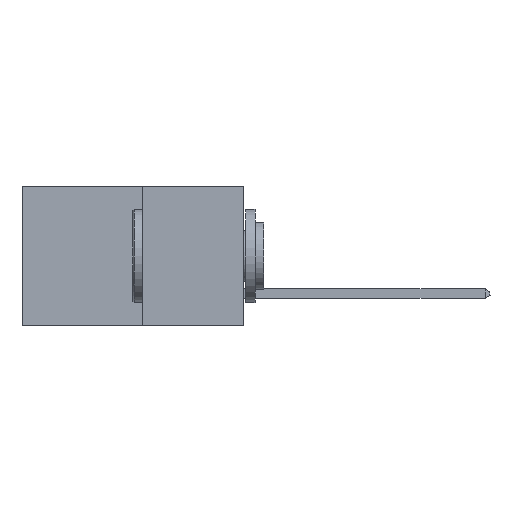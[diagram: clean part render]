
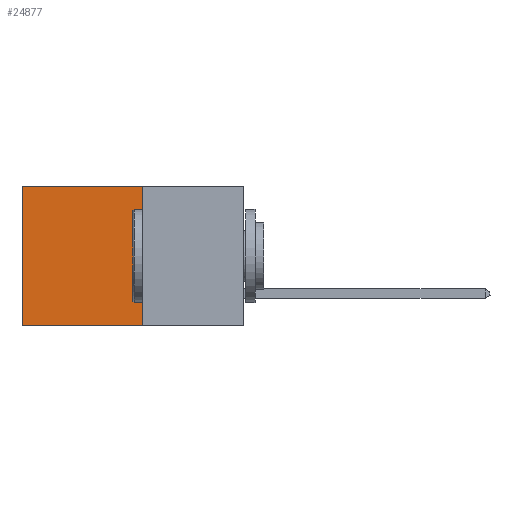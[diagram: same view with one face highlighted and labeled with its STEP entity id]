
A CAD part, left-side view. The second image highlights one B-rep face of the part: STEP entity #24877.
In plain terms, the highlighted planar face has unit normal (-1, 0, 0).
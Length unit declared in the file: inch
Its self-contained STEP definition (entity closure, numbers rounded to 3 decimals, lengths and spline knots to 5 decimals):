
#462 = ORIENTED_EDGE ( 'NONE', *, *, #16358, .F. ) ;
#655 = AXIS2_PLACEMENT_3D ( 'NONE', #19266, #4052, #21832 ) ;
#2775 = VERTEX_POINT ( 'NONE', #30983 ) ;
#2862 = CARTESIAN_POINT ( 'NONE',  ( 0.277, 0.59, 0. ) ) ;
#4052 = DIRECTION ( 'NONE',  ( 1., 0., 0. ) ) ;
#5058 = ORIENTED_EDGE ( 'NONE', *, *, #13953, .T. ) ;
#5789 = CARTESIAN_POINT ( 'NONE',  ( 0.277, 0.27, -0.37 ) ) ;
#6150 = EDGE_CURVE ( 'NONE', #16753, #2775, #8072, .T. ) ;
#6391 = LINE ( 'NONE', #27204, #19087 ) ;
#7884 = LINE ( 'NONE', #31618, #20602 ) ;
#8072 = LINE ( 'NONE', #5789, #27552 ) ;
#8224 = CARTESIAN_POINT ( 'NONE',  ( 0.277, 0.27, 0. ) ) ;
#9414 = DIRECTION ( 'NONE',  ( 0., 1., 0. ) ) ;
#9656 = EDGE_LOOP ( 'NONE', ( #11192, #462, #15031, #5058 ) ) ;
#11192 = ORIENTED_EDGE ( 'NONE', *, *, #12838, .T. ) ;
#12838 = EDGE_CURVE ( 'NONE', #27851, #20394, #7884, .T. ) ;
#13493 = CARTESIAN_POINT ( 'NONE',  ( 0.277, 0.59, -0.37 ) ) ;
#13953 = EDGE_CURVE ( 'NONE', #16753, #27851, #18541, .T. ) ;
#15031 = ORIENTED_EDGE ( 'NONE', *, *, #6150, .F. ) ;
#16086 = CARTESIAN_POINT ( 'NONE',  ( 0.277, 0.27, 0. ) ) ;
#16358 = EDGE_CURVE ( 'NONE', #2775, #20394, #6391, .T. ) ;
#16398 = DIRECTION ( 'NONE',  ( 0., 0., -1. ) ) ;
#16753 = VERTEX_POINT ( 'NONE', #16086 ) ;
#18541 = LINE ( 'NONE', #8224, #30426 ) ;
#19087 = VECTOR ( 'NONE', #9414, 39.37008 ) ;
#19266 = CARTESIAN_POINT ( 'NONE',  ( 0.277, 0.27, -0.37 ) ) ;
#20394 = VERTEX_POINT ( 'NONE', #13493 ) ;
#20602 = VECTOR ( 'NONE', #16398, 39.37008 ) ;
#21832 = DIRECTION ( 'NONE',  ( 0., 0., -1. ) ) ;
#24877 = ADVANCED_FACE ( 'NONE', ( #26883 ), #31959, .F. ) ;
#26883 = FACE_OUTER_BOUND ( 'NONE', #9656, .T. ) ;
#27204 = CARTESIAN_POINT ( 'NONE',  ( 0.277, 0.27, -0.37 ) ) ;
#27552 = VECTOR ( 'NONE', #28691, 39.37008 ) ;
#27851 = VERTEX_POINT ( 'NONE', #2862 ) ;
#28550 = DIRECTION ( 'NONE',  ( 0., 1., 0. ) ) ;
#28691 = DIRECTION ( 'NONE',  ( 0., 0., -1. ) ) ;
#30426 = VECTOR ( 'NONE', #28550, 39.37008 ) ;
#30983 = CARTESIAN_POINT ( 'NONE',  ( 0.277, 0.27, -0.37 ) ) ;
#31618 = CARTESIAN_POINT ( 'NONE',  ( 0.277, 0.59, -0.37 ) ) ;
#31959 = PLANE ( 'NONE',  #655 ) ;
